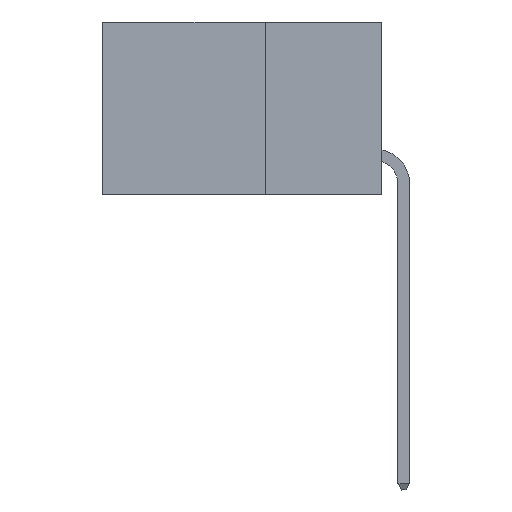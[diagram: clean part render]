
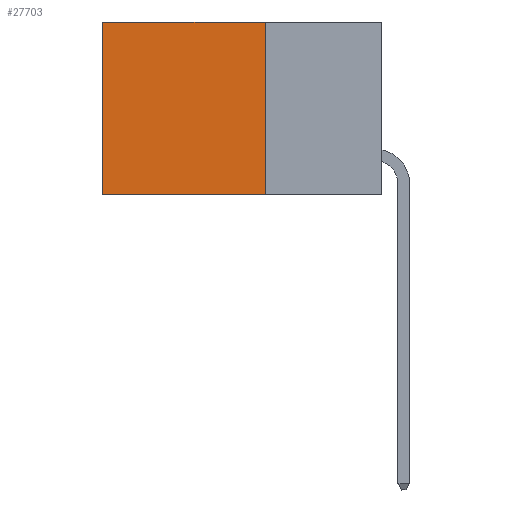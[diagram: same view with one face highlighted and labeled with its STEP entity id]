
A CAD part, left-side view. The second image highlights one B-rep face of the part: STEP entity #27703.
In plain terms, the highlighted planar face has unit normal (-1, 0, 0).
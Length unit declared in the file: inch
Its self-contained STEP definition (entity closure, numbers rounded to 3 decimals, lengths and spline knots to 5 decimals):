
#2151 = EDGE_CURVE ( 'NONE', #17773, #10171, #37772, .T. ) ;
#2367 = AXIS2_PLACEMENT_3D ( 'NONE', #32875, #3058, #14992 ) ;
#3058 = DIRECTION ( 'NONE',  ( 1., 0., 0. ) ) ;
#3690 = ORIENTED_EDGE ( 'NONE', *, *, #18798, .T. ) ;
#4726 = CARTESIAN_POINT ( 'NONE',  ( 0.2875, 0.25, -0.37 ) ) ;
#5522 = LINE ( 'NONE', #35143, #37552 ) ;
#6653 = EDGE_CURVE ( 'NONE', #10171, #13152, #23949, .T. ) ;
#7099 = CARTESIAN_POINT ( 'NONE',  ( 0.2875, 0.25, 0. ) ) ;
#7392 = EDGE_CURVE ( 'NONE', #17773, #18792, #18758, .T. ) ;
#8509 = CARTESIAN_POINT ( 'NONE',  ( 0.2875, 0.6, -0.37 ) ) ;
#10171 = VERTEX_POINT ( 'NONE', #4726 ) ;
#13152 = VERTEX_POINT ( 'NONE', #8509 ) ;
#13210 = DIRECTION ( 'NONE',  ( 0., 0., -1. ) ) ;
#14992 = DIRECTION ( 'NONE',  ( 0., 0., -1. ) ) ;
#17773 = VERTEX_POINT ( 'NONE', #7099 ) ;
#18758 = LINE ( 'NONE', #26780, #28546 ) ;
#18792 = VERTEX_POINT ( 'NONE', #25819 ) ;
#18798 = EDGE_CURVE ( 'NONE', #18792, #13152, #5522, .T. ) ;
#20894 = CARTESIAN_POINT ( 'NONE',  ( 0.2875, 0.25, -0.37 ) ) ;
#20938 = DIRECTION ( 'NONE',  ( 0., 1., 0. ) ) ;
#23949 = LINE ( 'NONE', #20894, #26728 ) ;
#24024 = DIRECTION ( 'NONE',  ( 0., 1., 0. ) ) ;
#24345 = FACE_OUTER_BOUND ( 'NONE', #34422, .T. ) ;
#24778 = VECTOR ( 'NONE', #13210, 39.37008 ) ;
#25819 = CARTESIAN_POINT ( 'NONE',  ( 0.2875, 0.6, 0. ) ) ;
#26728 = VECTOR ( 'NONE', #24024, 39.37008 ) ;
#26780 = CARTESIAN_POINT ( 'NONE',  ( 0.2875, 0.25, 0. ) ) ;
#26807 = PLANE ( 'NONE',  #2367 ) ;
#27703 = ADVANCED_FACE ( 'NONE', ( #24345 ), #26807, .F. ) ;
#28546 = VECTOR ( 'NONE', #20938, 39.37008 ) ;
#30184 = ORIENTED_EDGE ( 'NONE', *, *, #7392, .T. ) ;
#31766 = ORIENTED_EDGE ( 'NONE', *, *, #2151, .F. ) ;
#32225 = ORIENTED_EDGE ( 'NONE', *, *, #6653, .F. ) ;
#32875 = CARTESIAN_POINT ( 'NONE',  ( 0.2875, 0.25, 0. ) ) ;
#34422 = EDGE_LOOP ( 'NONE', ( #3690, #32225, #31766, #30184 ) ) ;
#35143 = CARTESIAN_POINT ( 'NONE',  ( 0.2875, 0.6, 0. ) ) ;
#37167 = CARTESIAN_POINT ( 'NONE',  ( 0.2875, 0.25, 0. ) ) ;
#37552 = VECTOR ( 'NONE', #38144, 39.37008 ) ;
#37772 = LINE ( 'NONE', #37167, #24778 ) ;
#38144 = DIRECTION ( 'NONE',  ( 0., 0., -1. ) ) ;
